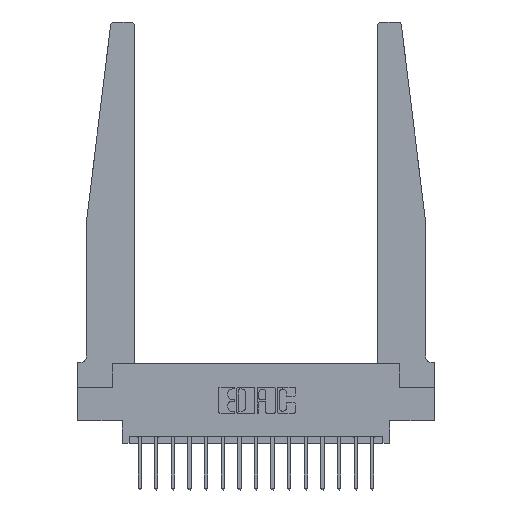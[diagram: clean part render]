
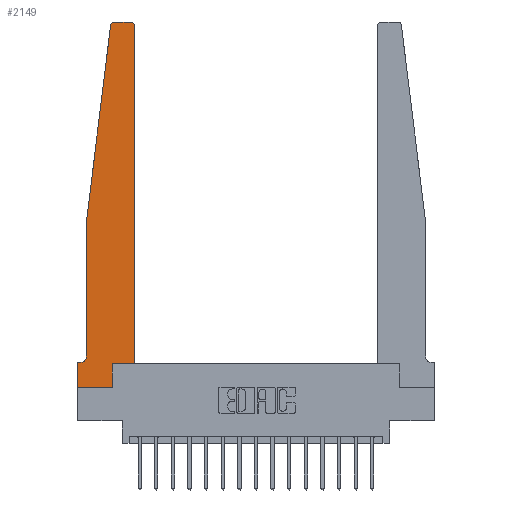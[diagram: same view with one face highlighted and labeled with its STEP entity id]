
A CAD part, top view. The second image highlights one B-rep face of the part: STEP entity #2149.
In plain terms, the highlighted planar face has unit normal (0, 0, 1).
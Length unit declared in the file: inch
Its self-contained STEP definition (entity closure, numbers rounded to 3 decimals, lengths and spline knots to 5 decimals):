
#6 = EDGE_LOOP ( 'NONE', ( #7773, #12816, #7984, #11213, #2793, #15476, #18036, #17749, #7718, #2519, #272, #15162 ) ) ;
#164 = VECTOR ( 'NONE', #5992, 39.37008 ) ;
#223 = CARTESIAN_POINT ( 'NONE',  ( 0.065, 1.25, 0.37 ) ) ;
#272 = ORIENTED_EDGE ( 'NONE', *, *, #17402, .T. ) ;
#638 = VERTEX_POINT ( 'NONE', #9882 ) ;
#1063 = EDGE_CURVE ( 'NONE', #13170, #16016, #12888, .T. ) ;
#1403 = LINE ( 'NONE', #5822, #12314 ) ;
#1784 = EDGE_CURVE ( 'NONE', #638, #15419, #10214, .T. ) ;
#1889 = AXIS2_PLACEMENT_3D ( 'NONE', #12217, #3706, #13632 ) ;
#2023 = DIRECTION ( 'NONE',  ( 0., 0., 1. ) ) ;
#2149 = ADVANCED_FACE ( 'NONE', ( #11079 ), #3350, .T. ) ;
#2179 = EDGE_CURVE ( 'NONE', #15419, #4673, #6441, .T. ) ;
#2308 = CIRCLE ( 'NONE', #17573, 0.03 ) ;
#2312 = DIRECTION ( 'NONE',  ( 0., -1., 0. ) ) ;
#2519 = ORIENTED_EDGE ( 'NONE', *, *, #9403, .T. ) ;
#2669 = DIRECTION ( 'NONE',  ( 1., 0., 0. ) ) ;
#2793 = ORIENTED_EDGE ( 'NONE', *, *, #13709, .T. ) ;
#2814 = DIRECTION ( 'NONE',  ( -0.122, -0.992, 0. ) ) ;
#2867 = CARTESIAN_POINT ( 'NONE',  ( 0.065, 0.2375, 0.37 ) ) ;
#3091 = DIRECTION ( 'NONE',  ( 1., 0., 0. ) ) ;
#3281 = DIRECTION ( 'NONE',  ( 0., 1., 0. ) ) ;
#3350 = PLANE ( 'NONE',  #8337 ) ;
#3629 = LINE ( 'NONE', #5107, #18251 ) ;
#3706 = DIRECTION ( 'NONE',  ( 0., 0., -1. ) ) ;
#4336 = CARTESIAN_POINT ( 'NONE',  ( 0.24675, 2.72367, 0.37 ) ) ;
#4611 = CARTESIAN_POINT ( 'NONE',  ( 0.015, 0.1875, 0.37 ) ) ;
#4673 = VERTEX_POINT ( 'NONE', #4336 ) ;
#4776 = DIRECTION ( 'NONE',  ( 1., 0., 0. ) ) ;
#5107 = CARTESIAN_POINT ( 'NONE',  ( 0., 0., 0.37 ) ) ;
#5117 = VECTOR ( 'NONE', #3091, 39.37008 ) ;
#5182 = VERTEX_POINT ( 'NONE', #223 ) ;
#5340 = VECTOR ( 'NONE', #3281, 39.37008 ) ;
#5822 = CARTESIAN_POINT ( 'NONE',  ( 0.425, 0.18, 0.37 ) ) ;
#5992 = DIRECTION ( 'NONE',  ( 0., -1., 0. ) ) ;
#6179 = CARTESIAN_POINT ( 'NONE',  ( 0., 0.1875, 0.37 ) ) ;
#6356 = CARTESIAN_POINT ( 'NONE',  ( 0.27653, 2.72, 0.37 ) ) ;
#6441 = CIRCLE ( 'NONE', #9298, 0.03 ) ;
#6489 = VECTOR ( 'NONE', #2669, 39.37008 ) ;
#6534 = DIRECTION ( 'NONE',  ( -1., 0., 0. ) ) ;
#6769 = EDGE_CURVE ( 'NONE', #10900, #17808, #7669, .T. ) ;
#6924 = VECTOR ( 'NONE', #8191, 39.37008 ) ;
#7018 = VERTEX_POINT ( 'NONE', #2867 ) ;
#7036 = CARTESIAN_POINT ( 'NONE',  ( 0., 0., 0.37 ) ) ;
#7277 = DIRECTION ( 'NONE',  ( 0., 1., 0. ) ) ;
#7669 = LINE ( 'NONE', #12161, #14707 ) ;
#7718 = ORIENTED_EDGE ( 'NONE', *, *, #1063, .T. ) ;
#7773 = ORIENTED_EDGE ( 'NONE', *, *, #1784, .T. ) ;
#7807 = DIRECTION ( 'NONE',  ( 1., 0., 0. ) ) ;
#7984 = ORIENTED_EDGE ( 'NONE', *, *, #12572, .T. ) ;
#8191 = DIRECTION ( 'NONE',  ( -1., 0., 0. ) ) ;
#8292 = CARTESIAN_POINT ( 'NONE',  ( 0.2605, 0.18, 0.37 ) ) ;
#8337 = AXIS2_PLACEMENT_3D ( 'NONE', #6179, #13282, #4776 ) ;
#8658 = LINE ( 'NONE', #18309, #11972 ) ;
#9263 = CARTESIAN_POINT ( 'NONE',  ( 0.425, 2.72, 0.37 ) ) ;
#9298 = AXIS2_PLACEMENT_3D ( 'NONE', #6356, #16231, #7807 ) ;
#9403 = EDGE_CURVE ( 'NONE', #16016, #14939, #15968, .T. ) ;
#9882 = CARTESIAN_POINT ( 'NONE',  ( 0.395, 2.75, 0.37 ) ) ;
#10214 = LINE ( 'NONE', #18041, #6924 ) ;
#10431 = VERTEX_POINT ( 'NONE', #9263 ) ;
#10463 = LINE ( 'NONE', #14438, #164 ) ;
#10550 = CARTESIAN_POINT ( 'NONE',  ( 0.395, 2.72, 0.37 ) ) ;
#10811 = CARTESIAN_POINT ( 'NONE',  ( 0.2605, 0., 0.37 ) ) ;
#10900 = VERTEX_POINT ( 'NONE', #4611 ) ;
#11079 = FACE_OUTER_BOUND ( 'NONE', #6, .T. ) ;
#11206 = EDGE_CURVE ( 'NONE', #12508, #13170, #17748, .T. ) ;
#11213 = ORIENTED_EDGE ( 'NONE', *, *, #11430, .T. ) ;
#11430 = EDGE_CURVE ( 'NONE', #5182, #7018, #10463, .T. ) ;
#11466 = CARTESIAN_POINT ( 'NONE',  ( 0.2605, 0.18, 0.37 ) ) ;
#11972 = VECTOR ( 'NONE', #2814, 39.37008 ) ;
#11973 = DIRECTION ( 'NONE',  ( 1., 0., 0. ) ) ;
#12149 = CIRCLE ( 'NONE', #1889, 0.05 ) ;
#12161 = CARTESIAN_POINT ( 'NONE',  ( 0.065, 0.1875, 0.37 ) ) ;
#12217 = CARTESIAN_POINT ( 'NONE',  ( 0.015, 0.2375, 0.37 ) ) ;
#12314 = VECTOR ( 'NONE', #7277, 39.37008 ) ;
#12508 = VERTEX_POINT ( 'NONE', #7036 ) ;
#12572 = EDGE_CURVE ( 'NONE', #4673, #5182, #8658, .T. ) ;
#12589 = CARTESIAN_POINT ( 'NONE',  ( 0.425, 0.18, 0.37 ) ) ;
#12816 = ORIENTED_EDGE ( 'NONE', *, *, #2179, .T. ) ;
#12888 = LINE ( 'NONE', #11466, #5340 ) ;
#13170 = VERTEX_POINT ( 'NONE', #10811 ) ;
#13282 = DIRECTION ( 'NONE',  ( 0., 0., 1. ) ) ;
#13632 = DIRECTION ( 'NONE',  ( -1., 0., 0. ) ) ;
#13709 = EDGE_CURVE ( 'NONE', #7018, #10900, #12149, .T. ) ;
#13841 = CARTESIAN_POINT ( 'NONE',  ( 0., 0.1875, 0.37 ) ) ;
#14438 = CARTESIAN_POINT ( 'NONE',  ( 0.065, 1.25, 0.37 ) ) ;
#14707 = VECTOR ( 'NONE', #6534, 39.37008 ) ;
#14939 = VERTEX_POINT ( 'NONE', #12589 ) ;
#15162 = ORIENTED_EDGE ( 'NONE', *, *, #15335, .T. ) ;
#15335 = EDGE_CURVE ( 'NONE', #10431, #638, #2308, .T. ) ;
#15419 = VERTEX_POINT ( 'NONE', #16344 ) ;
#15476 = ORIENTED_EDGE ( 'NONE', *, *, #6769, .T. ) ;
#15968 = LINE ( 'NONE', #17275, #5117 ) ;
#16016 = VERTEX_POINT ( 'NONE', #8292 ) ;
#16231 = DIRECTION ( 'NONE',  ( 0., 0., 1. ) ) ;
#16344 = CARTESIAN_POINT ( 'NONE',  ( 0.27653, 2.75, 0.37 ) ) ;
#17275 = CARTESIAN_POINT ( 'NONE',  ( 0.425, 0.18, 0.37 ) ) ;
#17402 = EDGE_CURVE ( 'NONE', #14939, #10431, #1403, .T. ) ;
#17573 = AXIS2_PLACEMENT_3D ( 'NONE', #10550, #2023, #11973 ) ;
#17700 = EDGE_CURVE ( 'NONE', #17808, #12508, #3629, .T. ) ;
#17748 = LINE ( 'NONE', #18228, #6489 ) ;
#17749 = ORIENTED_EDGE ( 'NONE', *, *, #11206, .T. ) ;
#17808 = VERTEX_POINT ( 'NONE', #13841 ) ;
#18036 = ORIENTED_EDGE ( 'NONE', *, *, #17700, .T. ) ;
#18041 = CARTESIAN_POINT ( 'NONE',  ( 0.25, 2.75, 0.37 ) ) ;
#18228 = CARTESIAN_POINT ( 'NONE',  ( 0., 0., 0.37 ) ) ;
#18251 = VECTOR ( 'NONE', #2312, 39.37008 ) ;
#18309 = CARTESIAN_POINT ( 'NONE',  ( 0.065, 1.25, 0.37 ) ) ;
